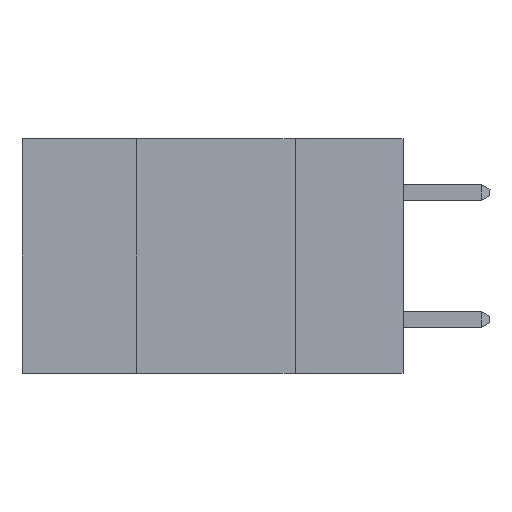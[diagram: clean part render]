
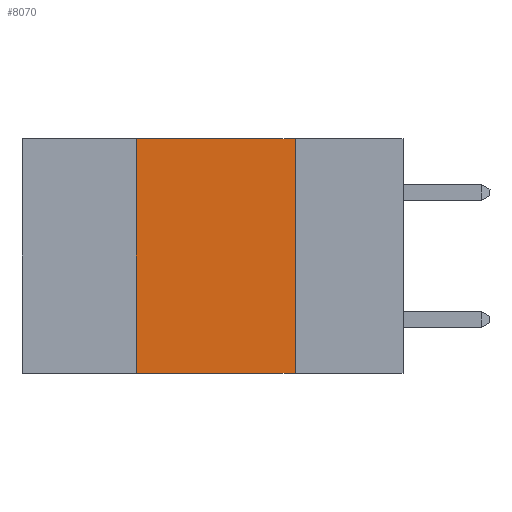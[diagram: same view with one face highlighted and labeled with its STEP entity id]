
A CAD part, left-side view. The second image highlights one B-rep face of the part: STEP entity #8070.
In plain terms, the highlighted planar face has unit normal (-1, 0, 0).
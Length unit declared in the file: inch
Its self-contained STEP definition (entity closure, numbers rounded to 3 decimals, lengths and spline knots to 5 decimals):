
#211 = DIRECTION ( 'NONE',  ( 0., -1., 0. ) ) ;
#239 = CARTESIAN_POINT ( 'NONE',  ( 0., 0.42, 0. ) ) ;
#350 = EDGE_CURVE ( 'NONE', #5072, #2154, #8213, .T. ) ;
#639 = LINE ( 'NONE', #7684, #9067 ) ;
#1167 = ORIENTED_EDGE ( 'NONE', *, *, #4191, .F. ) ;
#1195 = EDGE_LOOP ( 'NONE', ( #1167, #2899, #6104, #3473 ) ) ;
#2067 = VERTEX_POINT ( 'NONE', #239 ) ;
#2154 = VERTEX_POINT ( 'NONE', #9537 ) ;
#2428 = VECTOR ( 'NONE', #211, 39.37008 ) ;
#2485 = EDGE_CURVE ( 'NONE', #2067, #8733, #6494, .T. ) ;
#2648 = CARTESIAN_POINT ( 'NONE',  ( 0., 0.17, 0. ) ) ;
#2664 = DIRECTION ( 'NONE',  ( 0., 0., -1. ) ) ;
#2899 = ORIENTED_EDGE ( 'NONE', *, *, #2485, .F. ) ;
#2934 = CARTESIAN_POINT ( 'NONE',  ( 0., 0.42, 0. ) ) ;
#3150 = AXIS2_PLACEMENT_3D ( 'NONE', #9367, #7803, #2664 ) ;
#3427 = VECTOR ( 'NONE', #3939, 39.37008 ) ;
#3473 = ORIENTED_EDGE ( 'NONE', *, *, #350, .T. ) ;
#3939 = DIRECTION ( 'NONE',  ( 0., 0., 1. ) ) ;
#4026 = DIRECTION ( 'NONE',  ( 0., 0., -1. ) ) ;
#4191 = EDGE_CURVE ( 'NONE', #8733, #2154, #639, .T. ) ;
#4852 = DIRECTION ( 'NONE',  ( 0., -1., 0. ) ) ;
#4946 = FACE_OUTER_BOUND ( 'NONE', #1195, .T. ) ;
#5072 = VERTEX_POINT ( 'NONE', #5812 ) ;
#5406 = CARTESIAN_POINT ( 'NONE',  ( 0., 0.6, 0. ) ) ;
#5812 = CARTESIAN_POINT ( 'NONE',  ( 0., 0.42, -0.37 ) ) ;
#6104 = ORIENTED_EDGE ( 'NONE', *, *, #8369, .F. ) ;
#6229 = VECTOR ( 'NONE', #4852, 39.37008 ) ;
#6358 = PLANE ( 'NONE',  #3150 ) ;
#6494 = LINE ( 'NONE', #5406, #2428 ) ;
#6911 = LINE ( 'NONE', #2934, #3427 ) ;
#7684 = CARTESIAN_POINT ( 'NONE',  ( 0., 0.17, 0. ) ) ;
#7803 = DIRECTION ( 'NONE',  ( 1., 0., 0. ) ) ;
#8070 = ADVANCED_FACE ( 'NONE', ( #4946 ), #6358, .F. ) ;
#8213 = LINE ( 'NONE', #9358, #6229 ) ;
#8369 = EDGE_CURVE ( 'NONE', #5072, #2067, #6911, .T. ) ;
#8733 = VERTEX_POINT ( 'NONE', #2648 ) ;
#9067 = VECTOR ( 'NONE', #4026, 39.37008 ) ;
#9358 = CARTESIAN_POINT ( 'NONE',  ( 0., 0.6, -0.37 ) ) ;
#9367 = CARTESIAN_POINT ( 'NONE',  ( 0., 0.6, 0. ) ) ;
#9537 = CARTESIAN_POINT ( 'NONE',  ( 0., 0.17, -0.37 ) ) ;
